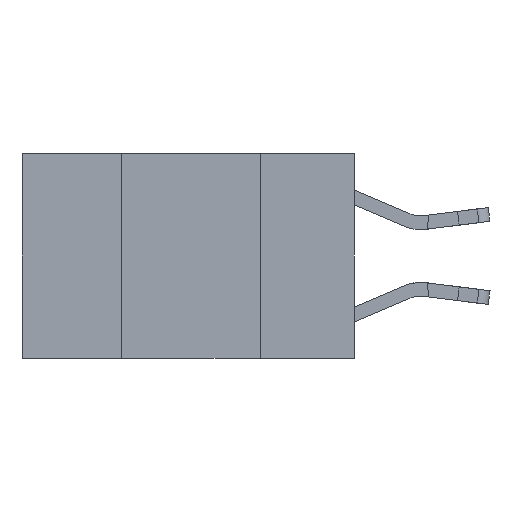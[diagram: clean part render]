
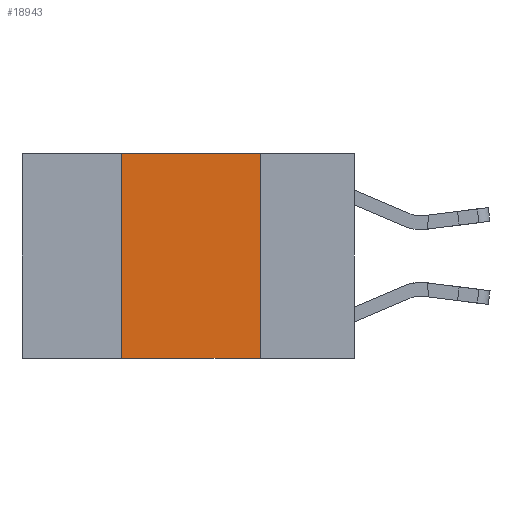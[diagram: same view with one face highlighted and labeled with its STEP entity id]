
A CAD part, left-side view. The second image highlights one B-rep face of the part: STEP entity #18943.
In plain terms, the highlighted planar face has unit normal (-1, 0, 0).
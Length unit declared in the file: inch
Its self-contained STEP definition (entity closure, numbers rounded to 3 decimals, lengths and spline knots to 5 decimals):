
#1209 = CARTESIAN_POINT ( 'NONE',  ( 0., 0.42, -0.37 ) ) ;
#2961 = ORIENTED_EDGE ( 'NONE', *, *, #5049, .F. ) ;
#3256 = LINE ( 'NONE', #15570, #20008 ) ;
#3442 = DIRECTION ( 'NONE',  ( 0., 0., 1. ) ) ;
#3471 = AXIS2_PLACEMENT_3D ( 'NONE', #3858, #15973, #5600 ) ;
#3858 = CARTESIAN_POINT ( 'NONE',  ( 0., 0.6, 0. ) ) ;
#5049 = EDGE_CURVE ( 'NONE', #14819, #11820, #7041, .T. ) ;
#5214 = DIRECTION ( 'NONE',  ( 0., -1., 0. ) ) ;
#5600 = DIRECTION ( 'NONE',  ( 0., 0., -1. ) ) ;
#6310 = DIRECTION ( 'NONE',  ( 0., 0., -1. ) ) ;
#7041 = LINE ( 'NONE', #17261, #20783 ) ;
#7550 = ORIENTED_EDGE ( 'NONE', *, *, #16851, .T. ) ;
#8922 = CARTESIAN_POINT ( 'NONE',  ( 0., 0.42, 0. ) ) ;
#10180 = EDGE_CURVE ( 'NONE', #13068, #11013, #15229, .T. ) ;
#11013 = VERTEX_POINT ( 'NONE', #20521 ) ;
#11086 = ORIENTED_EDGE ( 'NONE', *, *, #10180, .F. ) ;
#11664 = DIRECTION ( 'NONE',  ( 0., -1., 0. ) ) ;
#11710 = EDGE_CURVE ( 'NONE', #11820, #13068, #3256, .T. ) ;
#11820 = VERTEX_POINT ( 'NONE', #8922 ) ;
#11929 = VECTOR ( 'NONE', #11664, 39.37008 ) ;
#12909 = FACE_OUTER_BOUND ( 'NONE', #20466, .T. ) ;
#13068 = VERTEX_POINT ( 'NONE', #17183 ) ;
#14695 = VECTOR ( 'NONE', #6310, 39.37008 ) ;
#14819 = VERTEX_POINT ( 'NONE', #1209 ) ;
#15229 = LINE ( 'NONE', #18404, #14695 ) ;
#15570 = CARTESIAN_POINT ( 'NONE',  ( 0., 0.6, 0. ) ) ;
#15973 = DIRECTION ( 'NONE',  ( 1., 0., 0. ) ) ;
#16234 = ORIENTED_EDGE ( 'NONE', *, *, #11710, .F. ) ;
#16851 = EDGE_CURVE ( 'NONE', #14819, #11013, #21076, .T. ) ;
#17183 = CARTESIAN_POINT ( 'NONE',  ( 0., 0.17, 0. ) ) ;
#17261 = CARTESIAN_POINT ( 'NONE',  ( 0., 0.42, 0. ) ) ;
#18404 = CARTESIAN_POINT ( 'NONE',  ( 0., 0.17, 0. ) ) ;
#18943 = ADVANCED_FACE ( 'NONE', ( #12909 ), #21034, .F. ) ;
#20008 = VECTOR ( 'NONE', #5214, 39.37008 ) ;
#20255 = CARTESIAN_POINT ( 'NONE',  ( 0., 0.6, -0.37 ) ) ;
#20466 = EDGE_LOOP ( 'NONE', ( #11086, #16234, #2961, #7550 ) ) ;
#20521 = CARTESIAN_POINT ( 'NONE',  ( 0., 0.17, -0.37 ) ) ;
#20783 = VECTOR ( 'NONE', #3442, 39.37008 ) ;
#21034 = PLANE ( 'NONE',  #3471 ) ;
#21076 = LINE ( 'NONE', #20255, #11929 ) ;
